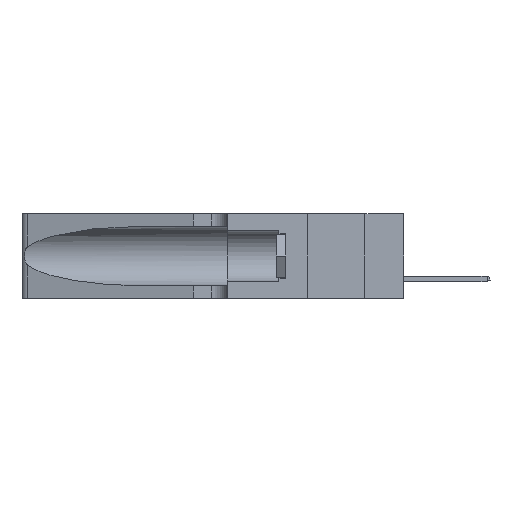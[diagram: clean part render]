
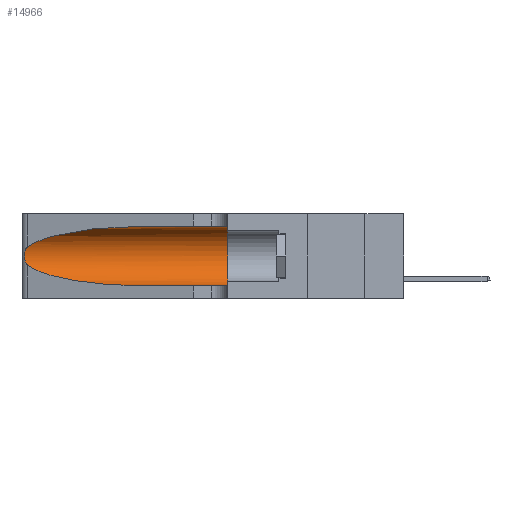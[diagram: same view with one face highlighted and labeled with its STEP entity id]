
A CAD part, left-side view. The second image highlights one B-rep face of the part: STEP entity #14966.
In plain terms, the highlighted cylindrical face has radius 3.308 mm (diameter 6.617 mm), a partial arc.
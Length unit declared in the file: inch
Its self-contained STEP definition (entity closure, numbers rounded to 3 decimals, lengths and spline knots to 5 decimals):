
#285 = AXIS2_PLACEMENT_3D ( 'NONE', #10859, #17200, #5614 ) ;
#357 = VECTOR ( 'NONE', #15864, 39.37008 ) ;
#439 =( BOUNDED_CURVE ( )  B_SPLINE_CURVE ( 3, ( #17775, #2852, #12873, #20945 ),
 .UNSPECIFIED., .F., .T. ) 
 B_SPLINE_CURVE_WITH_KNOTS ( ( 4, 4 ),
 ( 1.5708, 2.84003 ),
 .UNSPECIFIED. ) 
 CURVE ( )  GEOMETRIC_REPRESENTATION_ITEM ( )  RATIONAL_B_SPLINE_CURVE ( ( 1., 0.87, 0.87, 1. ) ) 
 REPRESENTATION_ITEM ( '' )  );
#671 = ORIENTED_EDGE ( 'NONE', *, *, #13111, .T. ) ;
#997 = DIRECTION ( 'NONE',  ( 0., 1., 0. ) ) ;
#1099 = CARTESIAN_POINT ( 'NONE',  ( 0.25487, 1.22718, 0.14631 ) ) ;
#1127 = CARTESIAN_POINT ( 'NONE',  ( 0.25487, 1.22718, 0.14631 ) ) ;
#1677 = ORIENTED_EDGE ( 'NONE', *, *, #17058, .T. ) ;
#2354 = CIRCLE ( 'NONE', #4276, 0.13025 ) ;
#2679 = CARTESIAN_POINT ( 'NONE',  ( 0.2373, 1.15595, 0.08982 ) ) ;
#2749 = CARTESIAN_POINT ( 'NONE',  ( 0.1305, 0.72297, 0.05475 ) ) ;
#2852 = CARTESIAN_POINT ( 'NONE',  ( 0.18966, 0.96281, 0.31525 ) ) ;
#3689 = VERTEX_POINT ( 'NONE', #21403 ) ;
#3969 = CARTESIAN_POINT ( 'NONE',  ( 0.1305, 0.35, 0.31525 ) ) ;
#4228 = CARTESIAN_POINT ( 'NONE',  ( 0.1305, 0.35, 0.185 ) ) ;
#4276 = AXIS2_PLACEMENT_3D ( 'NONE', #4228, #997, #10788 ) ;
#4464 = CARTESIAN_POINT ( 'NONE',  ( 0.25639, 1.23184, 0.21858 ) ) ;
#4542 = CARTESIAN_POINT ( 'NONE',  ( 0.26075, 1.23896, 0.19203 ) ) ;
#4889 = VERTEX_POINT ( 'NONE', #3969 ) ;
#5453 = VECTOR ( 'NONE', #7664, 39.37008 ) ;
#5614 = DIRECTION ( 'NONE',  ( 0., 0., -1. ) ) ;
#5762 = VERTEX_POINT ( 'NONE', #18314 ) ;
#5796 = EDGE_CURVE ( 'NONE', #3689, #8728, #16406, .T. ) ;
#6097 = CARTESIAN_POINT ( 'NONE',  ( 0.25487, 1.22718, 0.14631 ) ) ;
#6277 = FACE_OUTER_BOUND ( 'NONE', #7511, .T. ) ;
#7511 = EDGE_LOOP ( 'NONE', ( #671, #1677, #10609, #20433, #17634, #20974 ) ) ;
#7664 = DIRECTION ( 'NONE',  ( 0., -1., 0. ) ) ;
#7830 = CARTESIAN_POINT ( 'NONE',  ( 0.25555, 1.22994, 0.2215 ) ) ;
#7910 = CARTESIAN_POINT ( 'NONE',  ( 0.1305, 0.72297, 0.31525 ) ) ;
#7936 = CARTESIAN_POINT ( 'NONE',  ( 0.1305, 1.61858, 0.05475 ) ) ;
#8002 = VERTEX_POINT ( 'NONE', #1127 ) ;
#8728 = VERTEX_POINT ( 'NONE', #19649 ) ;
#9446 = CARTESIAN_POINT ( 'NONE',  ( 0.26017, 1.23833, 0.17102 ) ) ;
#10609 = ORIENTED_EDGE ( 'NONE', *, *, #20171, .T. ) ;
#10788 = DIRECTION ( 'NONE',  ( 0., 0., 1. ) ) ;
#10859 = CARTESIAN_POINT ( 'NONE',  ( 0.1305, 1.61858, 0.185 ) ) ;
#11180 = CARTESIAN_POINT ( 'NONE',  ( 0.25639, 1.23186, 0.15144 ) ) ;
#12010 = EDGE_CURVE ( 'NONE', #4889, #8728, #2354, .T. ) ;
#12495 = CARTESIAN_POINT ( 'NONE',  ( 0.1305, 1.61858, 0.31525 ) ) ;
#12788 = CARTESIAN_POINT ( 'NONE',  ( 0.25555, 1.22993, 0.14849 ) ) ;
#12873 = CARTESIAN_POINT ( 'NONE',  ( 0.2373, 1.15595, 0.28018 ) ) ;
#13071 = LINE ( 'NONE', #12495, #357 ) ;
#13111 = EDGE_CURVE ( 'NONE', #16541, #5762, #439, .T. ) ;
#13865 =( BOUNDED_CURVE ( )  B_SPLINE_CURVE ( 3, ( #1099, #2679, #14155, #2749 ),
 .UNSPECIFIED., .F., .T. ) 
 B_SPLINE_CURVE_WITH_KNOTS ( ( 4, 4 ),
 ( 3.44316, 4.71239 ),
 .UNSPECIFIED. ) 
 CURVE ( )  GEOMETRIC_REPRESENTATION_ITEM ( )  RATIONAL_B_SPLINE_CURVE ( ( 1., 0.87, 0.87, 1. ) ) 
 REPRESENTATION_ITEM ( '' )  );
#14155 = CARTESIAN_POINT ( 'NONE',  ( 0.18966, 0.96281, 0.05475 ) ) ;
#14394 = EDGE_CURVE ( 'NONE', #16541, #4889, #13071, .T. ) ;
#14600 = CYLINDRICAL_SURFACE ( 'NONE', #285, 0.13025 ) ;
#14655 = CARTESIAN_POINT ( 'NONE',  ( 0.25854, 1.2359, 0.20912 ) ) ;
#14790 = B_SPLINE_CURVE_WITH_KNOTS ( 'NONE', 3,
 ( #19444, #7830, #4464, #21171, #14655, #17817, #4542, #21242, #9446, #19720, #16151, #11180, #12788, #6097 ),
 .UNSPECIFIED., .F., .F.,
 ( 4, 2, 2, 2, 2, 2, 4 ),
 ( 0., 0.00027, 0.00053, 0.00107, 0.0016, 0.00187, 0.00214 ),
 .UNSPECIFIED. ) ;
#14966 = ADVANCED_FACE ( 'NONE', ( #6277 ), #14600, .F. ) ;
#15864 = DIRECTION ( 'NONE',  ( 0., -1., 0. ) ) ;
#16151 = CARTESIAN_POINT ( 'NONE',  ( 0.25789, 1.23486, 0.15765 ) ) ;
#16406 = LINE ( 'NONE', #7936, #5453 ) ;
#16541 = VERTEX_POINT ( 'NONE', #7910 ) ;
#17058 = EDGE_CURVE ( 'NONE', #5762, #8002, #14790, .T. ) ;
#17200 = DIRECTION ( 'NONE',  ( 0., -1., 0. ) ) ;
#17634 = ORIENTED_EDGE ( 'NONE', *, *, #12010, .F. ) ;
#17775 = CARTESIAN_POINT ( 'NONE',  ( 0.1305, 0.72297, 0.31525 ) ) ;
#17817 = CARTESIAN_POINT ( 'NONE',  ( 0.26018, 1.23835, 0.19895 ) ) ;
#18314 = CARTESIAN_POINT ( 'NONE',  ( 0.25487, 1.22718, 0.22369 ) ) ;
#19444 = CARTESIAN_POINT ( 'NONE',  ( 0.25487, 1.22718, 0.22369 ) ) ;
#19649 = CARTESIAN_POINT ( 'NONE',  ( 0.1305, 0.35, 0.05475 ) ) ;
#19720 = CARTESIAN_POINT ( 'NONE',  ( 0.25856, 1.23593, 0.16098 ) ) ;
#20171 = EDGE_CURVE ( 'NONE', #8002, #3689, #13865, .T. ) ;
#20433 = ORIENTED_EDGE ( 'NONE', *, *, #5796, .T. ) ;
#20945 = CARTESIAN_POINT ( 'NONE',  ( 0.25487, 1.22718, 0.22369 ) ) ;
#20974 = ORIENTED_EDGE ( 'NONE', *, *, #14394, .F. ) ;
#21171 = CARTESIAN_POINT ( 'NONE',  ( 0.25787, 1.23484, 0.2124 ) ) ;
#21242 = CARTESIAN_POINT ( 'NONE',  ( 0.26075, 1.23896, 0.178 ) ) ;
#21403 = CARTESIAN_POINT ( 'NONE',  ( 0.1305, 0.72297, 0.05475 ) ) ;
